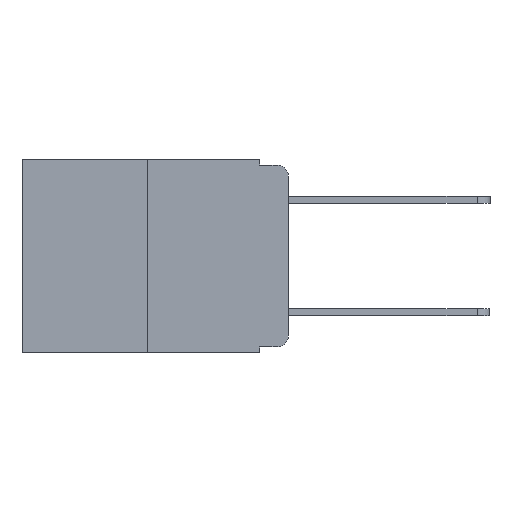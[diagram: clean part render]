
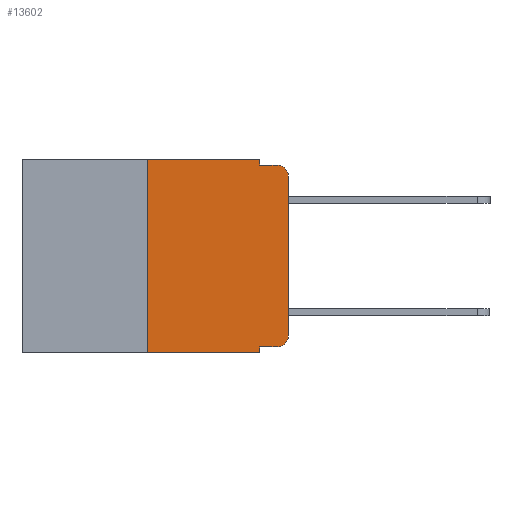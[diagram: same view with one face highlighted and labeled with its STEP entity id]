
A CAD part, left-side view. The second image highlights one B-rep face of the part: STEP entity #13602.
In plain terms, the highlighted planar face has unit normal (-1, 0, 0).
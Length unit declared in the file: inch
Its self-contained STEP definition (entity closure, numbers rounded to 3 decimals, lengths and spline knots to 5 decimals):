
#332 = CIRCLE ( 'NONE', #13824, 0.02 ) ;
#1074 = ORIENTED_EDGE ( 'NONE', *, *, #9953, .T. ) ;
#1084 = CARTESIAN_POINT ( 'NONE',  ( 0., 0.25, -0.343 ) ) ;
#1096 = EDGE_CURVE ( 'NONE', #6155, #5839, #5736, .T. ) ;
#1129 = CARTESIAN_POINT ( 'NONE',  ( 0., 0.25, 0. ) ) ;
#1329 = FACE_OUTER_BOUND ( 'NONE', #1470, .T. ) ;
#1470 = EDGE_LOOP ( 'NONE', ( #1074, #9353, #15327, #5768, #13806, #18350, #8007, #13592, #10730, #2539 ) ) ;
#1471 = VECTOR ( 'NONE', #12742, 39.37008 ) ;
#1485 = VERTEX_POINT ( 'NONE', #5277 ) ;
#1741 = VECTOR ( 'NONE', #7306, 39.37008 ) ;
#2080 = VERTEX_POINT ( 'NONE', #7954 ) ;
#2446 = CARTESIAN_POINT ( 'NONE',  ( 0., 0., -0.313 ) ) ;
#2482 = VECTOR ( 'NONE', #6620, 39.37008 ) ;
#2484 = VECTOR ( 'NONE', #13429, 39.37008 ) ;
#2539 = ORIENTED_EDGE ( 'NONE', *, *, #11623, .T. ) ;
#2884 = CARTESIAN_POINT ( 'NONE',  ( 0., 0.051, -0.01 ) ) ;
#3056 = CARTESIAN_POINT ( 'NONE',  ( 0., 0.02, -0.313 ) ) ;
#3954 = LINE ( 'NONE', #14580, #7790 ) ;
#4486 = PLANE ( 'NONE',  #11371 ) ;
#4541 = DIRECTION ( 'NONE',  ( 0., 0., -1. ) ) ;
#4744 = DIRECTION ( 'NONE',  ( -1., 0., 0. ) ) ;
#5244 = VECTOR ( 'NONE', #11370, 39.37008 ) ;
#5277 = CARTESIAN_POINT ( 'NONE',  ( 0., 0.02, -0.333 ) ) ;
#5548 = CARTESIAN_POINT ( 'NONE',  ( 0., 0.473, 0. ) ) ;
#5736 = LINE ( 'NONE', #2884, #1741 ) ;
#5768 = ORIENTED_EDGE ( 'NONE', *, *, #17576, .F. ) ;
#5839 = VERTEX_POINT ( 'NONE', #18201 ) ;
#5883 = VERTEX_POINT ( 'NONE', #1084 ) ;
#5896 = EDGE_CURVE ( 'NONE', #17298, #2080, #16783, .T. ) ;
#5983 = DIRECTION ( 'NONE',  ( 0., 0., -1. ) ) ;
#6060 = DIRECTION ( 'NONE',  ( 0., -1., 0. ) ) ;
#6155 = VERTEX_POINT ( 'NONE', #14741 ) ;
#6413 = LINE ( 'NONE', #12311, #2482 ) ;
#6416 = LINE ( 'NONE', #10535, #2484 ) ;
#6620 = DIRECTION ( 'NONE',  ( 0., -1., 0. ) ) ;
#6690 = DIRECTION ( 'NONE',  ( 0., 0., -1. ) ) ;
#7306 = DIRECTION ( 'NONE',  ( 0., -1., 0. ) ) ;
#7607 = EDGE_CURVE ( 'NONE', #11135, #5839, #14754, .T. ) ;
#7673 = CARTESIAN_POINT ( 'NONE',  ( 0., 0., -0.03 ) ) ;
#7790 = VECTOR ( 'NONE', #6060, 39.37008 ) ;
#7954 = CARTESIAN_POINT ( 'NONE',  ( 0., 0.051, 0. ) ) ;
#8007 = ORIENTED_EDGE ( 'NONE', *, *, #12976, .T. ) ;
#8952 = CARTESIAN_POINT ( 'NONE',  ( 0., 0.25, 0. ) ) ;
#9080 = LINE ( 'NONE', #1129, #5244 ) ;
#9232 = VERTEX_POINT ( 'NONE', #11450 ) ;
#9353 = ORIENTED_EDGE ( 'NONE', *, *, #7607, .T. ) ;
#9599 = VECTOR ( 'NONE', #9743, 39.37008 ) ;
#9743 = DIRECTION ( 'NONE',  ( 0., 0., 1. ) ) ;
#9840 = CARTESIAN_POINT ( 'NONE',  ( 0., 0.051, -0.333 ) ) ;
#9953 = EDGE_CURVE ( 'NONE', #12735, #11135, #10045, .T. ) ;
#10045 = LINE ( 'NONE', #15340, #9599 ) ;
#10535 = CARTESIAN_POINT ( 'NONE',  ( 0., 0.051, 0. ) ) ;
#10600 = VECTOR ( 'NONE', #6690, 39.37008 ) ;
#10730 = ORIENTED_EDGE ( 'NONE', *, *, #11270, .T. ) ;
#11135 = VERTEX_POINT ( 'NONE', #7673 ) ;
#11270 = EDGE_CURVE ( 'NONE', #13396, #1485, #6413, .T. ) ;
#11370 = DIRECTION ( 'NONE',  ( 0., 0., 1. ) ) ;
#11371 = AXIS2_PLACEMENT_3D ( 'NONE', #13103, #14498, #5983 ) ;
#11450 = CARTESIAN_POINT ( 'NONE',  ( 0., 0.051, -0.343 ) ) ;
#11623 = EDGE_CURVE ( 'NONE', #1485, #12735, #332, .T. ) ;
#11964 = EDGE_CURVE ( 'NONE', #5883, #17298, #9080, .T. ) ;
#12170 = AXIS2_PLACEMENT_3D ( 'NONE', #13343, #4744, #14745 ) ;
#12311 = CARTESIAN_POINT ( 'NONE',  ( 0., 0.051, -0.333 ) ) ;
#12735 = VERTEX_POINT ( 'NONE', #2446 ) ;
#12742 = DIRECTION ( 'NONE',  ( 0., -1., 0. ) ) ;
#12976 = EDGE_CURVE ( 'NONE', #5883, #9232, #3954, .T. ) ;
#13103 = CARTESIAN_POINT ( 'NONE',  ( 0., 0.473, 0. ) ) ;
#13160 = DIRECTION ( 'NONE',  ( -1., 0., 0. ) ) ;
#13343 = CARTESIAN_POINT ( 'NONE',  ( 0., 0.02, -0.03 ) ) ;
#13396 = VERTEX_POINT ( 'NONE', #9840 ) ;
#13429 = DIRECTION ( 'NONE',  ( 0., 0., -1. ) ) ;
#13592 = ORIENTED_EDGE ( 'NONE', *, *, #15382, .F. ) ;
#13602 = ADVANCED_FACE ( 'NONE', ( #1329 ), #4486, .F. ) ;
#13806 = ORIENTED_EDGE ( 'NONE', *, *, #5896, .F. ) ;
#13824 = AXIS2_PLACEMENT_3D ( 'NONE', #3056, #13160, #4541 ) ;
#14498 = DIRECTION ( 'NONE',  ( 1., 0., 0. ) ) ;
#14580 = CARTESIAN_POINT ( 'NONE',  ( 0., 0.473, -0.343 ) ) ;
#14741 = CARTESIAN_POINT ( 'NONE',  ( 0., 0.051, -0.01 ) ) ;
#14745 = DIRECTION ( 'NONE',  ( 0., 0., -1. ) ) ;
#14754 = CIRCLE ( 'NONE', #12170, 0.02 ) ;
#15327 = ORIENTED_EDGE ( 'NONE', *, *, #1096, .F. ) ;
#15340 = CARTESIAN_POINT ( 'NONE',  ( 0., 0., 0. ) ) ;
#15382 = EDGE_CURVE ( 'NONE', #13396, #9232, #6416, .T. ) ;
#16783 = LINE ( 'NONE', #5548, #1471 ) ;
#17298 = VERTEX_POINT ( 'NONE', #8952 ) ;
#17576 = EDGE_CURVE ( 'NONE', #2080, #6155, #18040, .T. ) ;
#17976 = CARTESIAN_POINT ( 'NONE',  ( 0., 0.051, 0. ) ) ;
#18040 = LINE ( 'NONE', #17976, #10600 ) ;
#18201 = CARTESIAN_POINT ( 'NONE',  ( 0., 0.02, -0.01 ) ) ;
#18350 = ORIENTED_EDGE ( 'NONE', *, *, #11964, .F. ) ;
